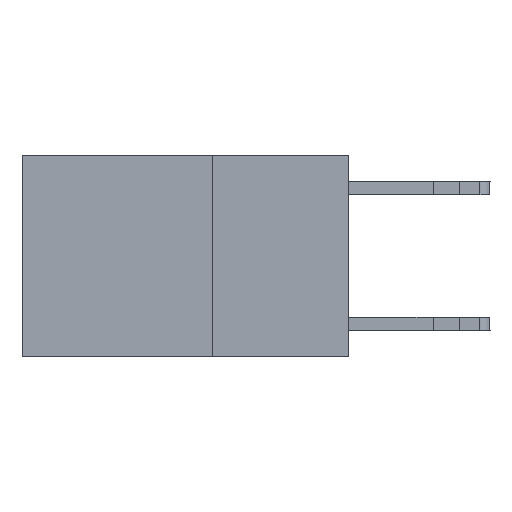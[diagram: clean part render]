
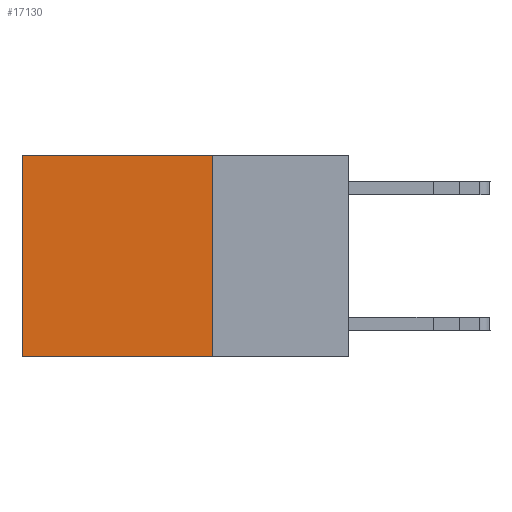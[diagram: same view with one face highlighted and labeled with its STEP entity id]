
A CAD part, left-side view. The second image highlights one B-rep face of the part: STEP entity #17130.
In plain terms, the highlighted planar face has unit normal (-1, 0, 0).
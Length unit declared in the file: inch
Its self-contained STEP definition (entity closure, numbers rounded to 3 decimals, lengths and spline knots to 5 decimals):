
#948 = DIRECTION ( 'NONE',  ( 0., 0., -1. ) ) ;
#1727 = CARTESIAN_POINT ( 'NONE',  ( 0.2625, 0.6, -0.37 ) ) ;
#1771 = VECTOR ( 'NONE', #7372, 39.37008 ) ;
#2193 = CARTESIAN_POINT ( 'NONE',  ( 0.2625, 0.25, -0.37 ) ) ;
#3717 = EDGE_CURVE ( 'NONE', #14635, #7376, #22425, .T. ) ;
#3729 = LINE ( 'NONE', #9234, #1771 ) ;
#4230 = CARTESIAN_POINT ( 'NONE',  ( 0.2625, 0.25, 0. ) ) ;
#4965 = EDGE_CURVE ( 'NONE', #14635, #14749, #3729, .T. ) ;
#5162 = VECTOR ( 'NONE', #11792, 39.37008 ) ;
#5631 = ORIENTED_EDGE ( 'NONE', *, *, #3717, .F. ) ;
#5882 = FACE_OUTER_BOUND ( 'NONE', #21137, .T. ) ;
#5907 = CARTESIAN_POINT ( 'NONE',  ( 0.2625, 0.25, -0.37 ) ) ;
#7372 = DIRECTION ( 'NONE',  ( 0., 1., 0. ) ) ;
#7376 = VERTEX_POINT ( 'NONE', #5907 ) ;
#9234 = CARTESIAN_POINT ( 'NONE',  ( 0.2625, 0.25, 0. ) ) ;
#10220 = DIRECTION ( 'NONE',  ( 0., 0., -1. ) ) ;
#10478 = DIRECTION ( 'NONE',  ( 0., 1., 0. ) ) ;
#11088 = ORIENTED_EDGE ( 'NONE', *, *, #16786, .T. ) ;
#11500 = VECTOR ( 'NONE', #10220, 39.37008 ) ;
#11792 = DIRECTION ( 'NONE',  ( 0., 0., -1. ) ) ;
#12991 = VECTOR ( 'NONE', #10478, 39.37008 ) ;
#14617 = VERTEX_POINT ( 'NONE', #1727 ) ;
#14635 = VERTEX_POINT ( 'NONE', #15653 ) ;
#14749 = VERTEX_POINT ( 'NONE', #18067 ) ;
#15096 = PLANE ( 'NONE',  #20470 ) ;
#15653 = CARTESIAN_POINT ( 'NONE',  ( 0.2625, 0.25, 0. ) ) ;
#16272 = EDGE_CURVE ( 'NONE', #7376, #14617, #16471, .T. ) ;
#16471 = LINE ( 'NONE', #2193, #12991 ) ;
#16579 = ORIENTED_EDGE ( 'NONE', *, *, #16272, .F. ) ;
#16786 = EDGE_CURVE ( 'NONE', #14749, #14617, #21210, .T. ) ;
#17130 = ADVANCED_FACE ( 'NONE', ( #5882 ), #15096, .F. ) ;
#18067 = CARTESIAN_POINT ( 'NONE',  ( 0.2625, 0.6, 0. ) ) ;
#19648 = ORIENTED_EDGE ( 'NONE', *, *, #4965, .T. ) ;
#20470 = AXIS2_PLACEMENT_3D ( 'NONE', #4230, #22121, #948 ) ;
#21137 = EDGE_LOOP ( 'NONE', ( #11088, #16579, #5631, #19648 ) ) ;
#21210 = LINE ( 'NONE', #22971, #11500 ) ;
#21961 = CARTESIAN_POINT ( 'NONE',  ( 0.2625, 0.25, 0. ) ) ;
#22121 = DIRECTION ( 'NONE',  ( 1., 0., 0. ) ) ;
#22425 = LINE ( 'NONE', #21961, #5162 ) ;
#22971 = CARTESIAN_POINT ( 'NONE',  ( 0.2625, 0.6, 0. ) ) ;
